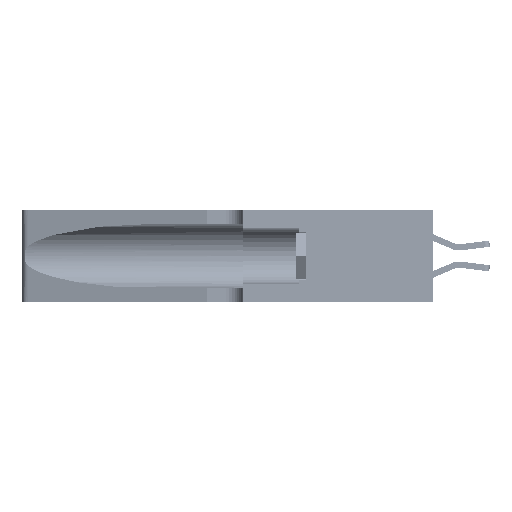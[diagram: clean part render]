
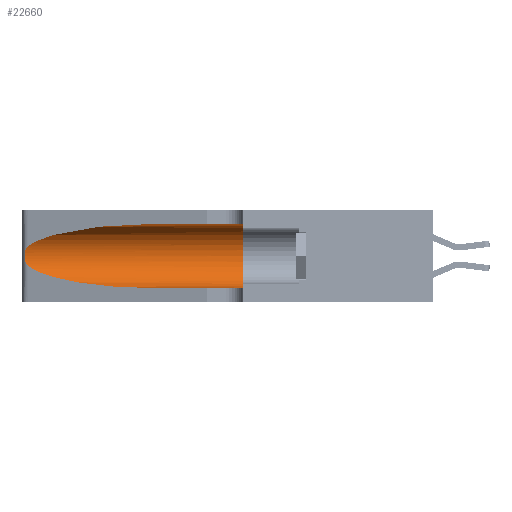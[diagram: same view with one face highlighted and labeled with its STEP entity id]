
A CAD part, left-side view. The second image highlights one B-rep face of the part: STEP entity #22660.
In plain terms, the highlighted cylindrical face has radius 3.308 mm (diameter 6.617 mm), a partial arc.
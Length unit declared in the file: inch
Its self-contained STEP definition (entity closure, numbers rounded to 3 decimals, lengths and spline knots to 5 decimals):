
#549 = CYLINDRICAL_SURFACE ( 'NONE', #12383, 0.13025 ) ;
#704 = LINE ( 'NONE', #51305, #34574 ) ;
#796 = CARTESIAN_POINT ( 'NONE',  ( 0.1305, 1.61858, 0.31525 ) ) ;
#1207 = CARTESIAN_POINT ( 'NONE',  ( 0.25789, 1.23486, 0.15765 ) ) ;
#1374 = CARTESIAN_POINT ( 'NONE',  ( 0.25856, 1.23593, 0.16098 ) ) ;
#2982 = CARTESIAN_POINT ( 'NONE',  ( 0.1305, 0.72297, 0.05475 ) ) ;
#3591 = ORIENTED_EDGE ( 'NONE', *, *, #43268, .T. ) ;
#3665 = DIRECTION ( 'NONE',  ( 0., -1., 0. ) ) ;
#4634 =( BOUNDED_CURVE ( )  B_SPLINE_CURVE ( 3, ( #8022, #51800, #31544, #28215 ),
 .UNSPECIFIED., .F., .F. ) 
 B_SPLINE_CURVE_WITH_KNOTS ( ( 4, 4 ),
 ( 1.5708, 2.84003 ),
 .UNSPECIFIED. ) 
 CURVE ( )  GEOMETRIC_REPRESENTATION_ITEM ( )  RATIONAL_B_SPLINE_CURVE ( ( 1., 0.87, 0.87, 1. ) ) 
 REPRESENTATION_ITEM ( '' )  );
#4940 = DIRECTION ( 'NONE',  ( 0., 1., 0. ) ) ;
#5041 = CARTESIAN_POINT ( 'NONE',  ( 0.25854, 1.2359, 0.20912 ) ) ;
#5126 = ORIENTED_EDGE ( 'NONE', *, *, #32593, .T. ) ;
#7043 = VERTEX_POINT ( 'NONE', #51378 ) ;
#7394 = FACE_OUTER_BOUND ( 'NONE', #46796, .T. ) ;
#7902 = CARTESIAN_POINT ( 'NONE',  ( 0.1305, 0.35, 0.05475 ) ) ;
#8022 = CARTESIAN_POINT ( 'NONE',  ( 0.1305, 0.72297, 0.31525 ) ) ;
#9053 = CARTESIAN_POINT ( 'NONE',  ( 0.26075, 1.23896, 0.178 ) ) ;
#9219 = CARTESIAN_POINT ( 'NONE',  ( 0.25487, 1.22718, 0.14631 ) ) ;
#9712 = CARTESIAN_POINT ( 'NONE',  ( 0.1305, 0.35, 0.31525 ) ) ;
#11266 = EDGE_CURVE ( 'NONE', #26675, #24179, #704, .T. ) ;
#11675 = B_SPLINE_CURVE_WITH_KNOTS ( 'NONE', 3,
 ( #17533, #17881, #25916, #45837, #5041, #25227, #33124, #9053, #37854, #1374, #1207, #41195, #37168, #9219 ),
 .UNSPECIFIED., .F., .F.,
 ( 4, 2, 2, 2, 2, 2, 4 ),
 ( 0., 0.00027, 0.00053, 0.00107, 0.0016, 0.00187, 0.00214 ),
 .UNSPECIFIED. ) ;
#12383 = AXIS2_PLACEMENT_3D ( 'NONE', #42597, #22644, #42099 ) ;
#16540 =( BOUNDED_CURVE ( )  B_SPLINE_CURVE ( 3, ( #23170, #27366, #51318, #2982 ),
 .UNSPECIFIED., .F., .F. ) 
 B_SPLINE_CURVE_WITH_KNOTS ( ( 4, 4 ),
 ( 3.44316, 4.71239 ),
 .UNSPECIFIED. ) 
 CURVE ( )  GEOMETRIC_REPRESENTATION_ITEM ( )  RATIONAL_B_SPLINE_CURVE ( ( 1., 0.87, 0.87, 1. ) ) 
 REPRESENTATION_ITEM ( '' )  );
#16718 = CARTESIAN_POINT ( 'NONE',  ( 0.1305, 0.35, 0.185 ) ) ;
#17533 = CARTESIAN_POINT ( 'NONE',  ( 0.25487, 1.22718, 0.22369 ) ) ;
#17881 = CARTESIAN_POINT ( 'NONE',  ( 0.25555, 1.22994, 0.2215 ) ) ;
#22644 = DIRECTION ( 'NONE',  ( 0., -1., 0. ) ) ;
#22660 = ADVANCED_FACE ( 'NONE', ( #7394 ), #549, .F. ) ;
#23170 = CARTESIAN_POINT ( 'NONE',  ( 0.25487, 1.22718, 0.14631 ) ) ;
#23788 = EDGE_CURVE ( 'NONE', #7043, #51308, #27365, .T. ) ;
#24179 = VERTEX_POINT ( 'NONE', #7902 ) ;
#25227 = CARTESIAN_POINT ( 'NONE',  ( 0.26018, 1.23835, 0.19895 ) ) ;
#25592 = CIRCLE ( 'NONE', #38820, 0.13025 ) ;
#25916 = CARTESIAN_POINT ( 'NONE',  ( 0.25639, 1.23184, 0.21858 ) ) ;
#26088 = ORIENTED_EDGE ( 'NONE', *, *, #26853, .F. ) ;
#26675 = VERTEX_POINT ( 'NONE', #36011 ) ;
#26853 = EDGE_CURVE ( 'NONE', #51308, #24179, #25592, .T. ) ;
#27365 = LINE ( 'NONE', #796, #47385 ) ;
#27366 = CARTESIAN_POINT ( 'NONE',  ( 0.2373, 1.15595, 0.08982 ) ) ;
#27959 = ORIENTED_EDGE ( 'NONE', *, *, #23788, .F. ) ;
#28215 = CARTESIAN_POINT ( 'NONE',  ( 0.25487, 1.22718, 0.22369 ) ) ;
#28978 = DIRECTION ( 'NONE',  ( 0., 0., 1. ) ) ;
#30180 = ORIENTED_EDGE ( 'NONE', *, *, #11266, .T. ) ;
#31544 = CARTESIAN_POINT ( 'NONE',  ( 0.2373, 1.15595, 0.28018 ) ) ;
#32277 = EDGE_CURVE ( 'NONE', #7043, #36786, #4634, .T. ) ;
#32593 = EDGE_CURVE ( 'NONE', #36786, #45000, #11675, .T. ) ;
#33052 = ORIENTED_EDGE ( 'NONE', *, *, #32277, .T. ) ;
#33124 = CARTESIAN_POINT ( 'NONE',  ( 0.26075, 1.23896, 0.19203 ) ) ;
#34574 = VECTOR ( 'NONE', #3665, 39.37008 ) ;
#36011 = CARTESIAN_POINT ( 'NONE',  ( 0.1305, 0.72297, 0.05475 ) ) ;
#36786 = VERTEX_POINT ( 'NONE', #44273 ) ;
#37168 = CARTESIAN_POINT ( 'NONE',  ( 0.25555, 1.22993, 0.14849 ) ) ;
#37854 = CARTESIAN_POINT ( 'NONE',  ( 0.26017, 1.23833, 0.17102 ) ) ;
#38664 = CARTESIAN_POINT ( 'NONE',  ( 0.25487, 1.22718, 0.14631 ) ) ;
#38820 = AXIS2_PLACEMENT_3D ( 'NONE', #16718, #4940, #28978 ) ;
#41195 = CARTESIAN_POINT ( 'NONE',  ( 0.25639, 1.23186, 0.15144 ) ) ;
#42099 = DIRECTION ( 'NONE',  ( 0., 0., -1. ) ) ;
#42597 = CARTESIAN_POINT ( 'NONE',  ( 0.1305, 1.61858, 0.185 ) ) ;
#43268 = EDGE_CURVE ( 'NONE', #45000, #26675, #16540, .T. ) ;
#44273 = CARTESIAN_POINT ( 'NONE',  ( 0.25487, 1.22718, 0.22369 ) ) ;
#45000 = VERTEX_POINT ( 'NONE', #38664 ) ;
#45448 = DIRECTION ( 'NONE',  ( 0., -1., 0. ) ) ;
#45837 = CARTESIAN_POINT ( 'NONE',  ( 0.25787, 1.23484, 0.2124 ) ) ;
#46796 = EDGE_LOOP ( 'NONE', ( #33052, #5126, #3591, #30180, #26088, #27959 ) ) ;
#47385 = VECTOR ( 'NONE', #45448, 39.37008 ) ;
#51305 = CARTESIAN_POINT ( 'NONE',  ( 0.1305, 1.61858, 0.05475 ) ) ;
#51308 = VERTEX_POINT ( 'NONE', #9712 ) ;
#51318 = CARTESIAN_POINT ( 'NONE',  ( 0.18966, 0.96281, 0.05475 ) ) ;
#51378 = CARTESIAN_POINT ( 'NONE',  ( 0.1305, 0.72297, 0.31525 ) ) ;
#51800 = CARTESIAN_POINT ( 'NONE',  ( 0.18966, 0.96281, 0.31525 ) ) ;
